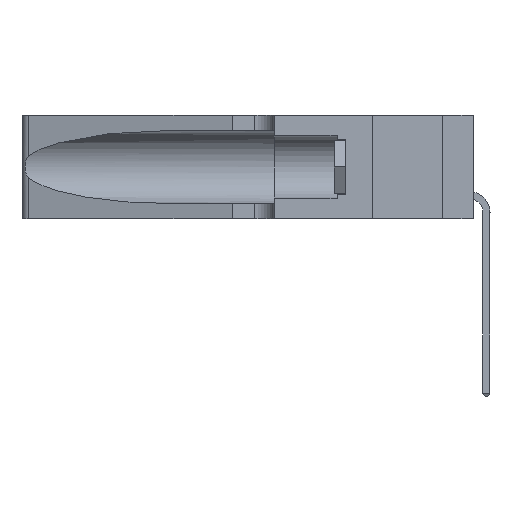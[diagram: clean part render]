
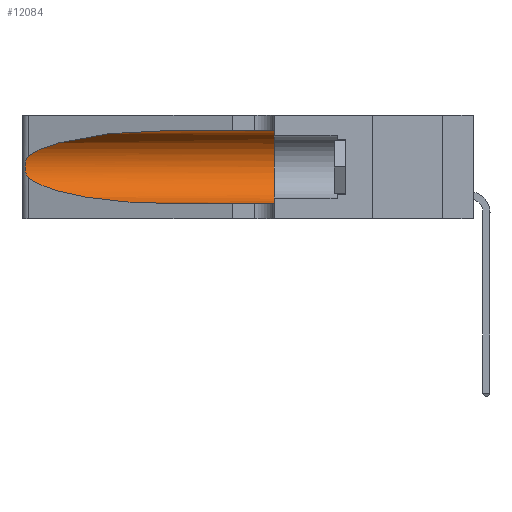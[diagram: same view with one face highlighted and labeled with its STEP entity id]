
A CAD part, left-side view. The second image highlights one B-rep face of the part: STEP entity #12084.
In plain terms, the highlighted cylindrical face has radius 3.308 mm (diameter 6.617 mm), a partial arc.
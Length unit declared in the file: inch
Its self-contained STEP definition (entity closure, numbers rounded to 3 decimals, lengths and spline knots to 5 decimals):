
#954 = CARTESIAN_POINT ( 'NONE',  ( 0.1305, 0.35, 0.185 ) ) ;
#1861 = EDGE_CURVE ( 'NONE', #3503, #39912, #5490, .T. ) ;
#1946 = VECTOR ( 'NONE', #24307, 39.37008 ) ;
#3069 = LINE ( 'NONE', #7002, #38445 ) ;
#3237 = VERTEX_POINT ( 'NONE', #25100 ) ;
#3428 = EDGE_CURVE ( 'NONE', #3237, #4760, #23144, .T. ) ;
#3503 = VERTEX_POINT ( 'NONE', #21320 ) ;
#4322 = AXIS2_PLACEMENT_3D ( 'NONE', #46529, #43051, #35353 ) ;
#4760 = VERTEX_POINT ( 'NONE', #31381 ) ;
#4955 = ORIENTED_EDGE ( 'NONE', *, *, #37876, .T. ) ;
#4978 = EDGE_CURVE ( 'NONE', #3503, #3237, #3069, .T. ) ;
#5490 =( BOUNDED_CURVE ( )  B_SPLINE_CURVE ( 3, ( #45179, #5866, #49540, #33863 ),
 .UNSPECIFIED., .F., .T. ) 
 B_SPLINE_CURVE_WITH_KNOTS ( ( 4, 4 ),
 ( 1.5708, 2.84003 ),
 .UNSPECIFIED. ) 
 CURVE ( )  GEOMETRIC_REPRESENTATION_ITEM ( )  RATIONAL_B_SPLINE_CURVE ( ( 1., 0.87, 0.87, 1. ) ) 
 REPRESENTATION_ITEM ( '' )  );
#5866 = CARTESIAN_POINT ( 'NONE',  ( 0.18966, 0.96281, 0.31525 ) ) ;
#6315 = CARTESIAN_POINT ( 'NONE',  ( 0.1305, 0.72297, 0.05475 ) ) ;
#6815 = CARTESIAN_POINT ( 'NONE',  ( 0.26075, 1.23896, 0.19203 ) ) ;
#7002 = CARTESIAN_POINT ( 'NONE',  ( 0.1305, 1.61858, 0.31525 ) ) ;
#8312 = EDGE_CURVE ( 'NONE', #39912, #24991, #38665, .T. ) ;
#10806 = CARTESIAN_POINT ( 'NONE',  ( 0.25487, 1.22718, 0.22369 ) ) ;
#10985 = CARTESIAN_POINT ( 'NONE',  ( 0.25854, 1.2359, 0.20912 ) ) ;
#12084 = ADVANCED_FACE ( 'NONE', ( #42642 ), #25212, .F. ) ;
#12540 = LINE ( 'NONE', #28469, #1946 ) ;
#13030 = AXIS2_PLACEMENT_3D ( 'NONE', #954, #40420, #17020 ) ;
#14125 = CARTESIAN_POINT ( 'NONE',  ( 0.25487, 1.22718, 0.14631 ) ) ;
#14796 = CARTESIAN_POINT ( 'NONE',  ( 0.25787, 1.23484, 0.2124 ) ) ;
#16387 = ORIENTED_EDGE ( 'NONE', *, *, #1861, .T. ) ;
#17020 = DIRECTION ( 'NONE',  ( 0., 0., 1. ) ) ;
#18325 = CARTESIAN_POINT ( 'NONE',  ( 0.2373, 1.15595, 0.08982 ) ) ;
#18797 = CARTESIAN_POINT ( 'NONE',  ( 0.25856, 1.23593, 0.16098 ) ) ;
#18806 = ORIENTED_EDGE ( 'NONE', *, *, #35010, .T. ) ;
#21320 = CARTESIAN_POINT ( 'NONE',  ( 0.1305, 0.72297, 0.31525 ) ) ;
#21759 = CARTESIAN_POINT ( 'NONE',  ( 0.25487, 1.22718, 0.14631 ) ) ;
#22218 = CARTESIAN_POINT ( 'NONE',  ( 0.25789, 1.23486, 0.15765 ) ) ;
#23144 = CIRCLE ( 'NONE', #13030, 0.13025 ) ;
#24307 = DIRECTION ( 'NONE',  ( 0., -1., 0. ) ) ;
#24991 = VERTEX_POINT ( 'NONE', #14125 ) ;
#25100 = CARTESIAN_POINT ( 'NONE',  ( 0.1305, 0.35, 0.31525 ) ) ;
#25212 = CYLINDRICAL_SURFACE ( 'NONE', #4322, 0.13025 ) ;
#25939 = CARTESIAN_POINT ( 'NONE',  ( 0.18966, 0.96281, 0.05475 ) ) ;
#26661 = DIRECTION ( 'NONE',  ( 0., -1., 0. ) ) ;
#26987 = EDGE_LOOP ( 'NONE', ( #16387, #29256, #4955, #18806, #27594, #30817 ) ) ;
#27594 = ORIENTED_EDGE ( 'NONE', *, *, #3428, .F. ) ;
#28469 = CARTESIAN_POINT ( 'NONE',  ( 0.1305, 1.61858, 0.05475 ) ) ;
#29256 = ORIENTED_EDGE ( 'NONE', *, *, #8312, .T. ) ;
#29987 = CARTESIAN_POINT ( 'NONE',  ( 0.1305, 0.72297, 0.05475 ) ) ;
#30817 = ORIENTED_EDGE ( 'NONE', *, *, #4978, .F. ) ;
#31381 = CARTESIAN_POINT ( 'NONE',  ( 0.1305, 0.35, 0.05475 ) ) ;
#33863 = CARTESIAN_POINT ( 'NONE',  ( 0.25487, 1.22718, 0.22369 ) ) ;
#33900 =( BOUNDED_CURVE ( )  B_SPLINE_CURVE ( 3, ( #21759, #18325, #25939, #29987 ),
 .UNSPECIFIED., .F., .F. ) 
 B_SPLINE_CURVE_WITH_KNOTS ( ( 4, 4 ),
 ( 3.44316, 4.71239 ),
 .UNSPECIFIED. ) 
 CURVE ( )  GEOMETRIC_REPRESENTATION_ITEM ( )  RATIONAL_B_SPLINE_CURVE ( ( 1., 0.87, 0.87, 1. ) ) 
 REPRESENTATION_ITEM ( '' )  );
#34408 = CARTESIAN_POINT ( 'NONE',  ( 0.26018, 1.23835, 0.19895 ) ) ;
#35010 = EDGE_CURVE ( 'NONE', #37280, #4760, #12540, .T. ) ;
#35353 = DIRECTION ( 'NONE',  ( 0., 0., -1. ) ) ;
#37280 = VERTEX_POINT ( 'NONE', #6315 ) ;
#37876 = EDGE_CURVE ( 'NONE', #24991, #37280, #33900, .T. ) ;
#38445 = VECTOR ( 'NONE', #26661, 39.37008 ) ;
#38535 = CARTESIAN_POINT ( 'NONE',  ( 0.25639, 1.23184, 0.21858 ) ) ;
#38665 = B_SPLINE_CURVE_WITH_KNOTS ( 'NONE', 3,
 ( #10806, #42652, #38535, #14796, #10985, #34408, #6815, #38709, #45933, #18797, #22218, #42292, #46116, #49898 ),
 .UNSPECIFIED., .F., .F.,
 ( 4, 2, 2, 2, 2, 2, 4 ),
 ( 0., 0.00027, 0.00053, 0.00107, 0.0016, 0.00187, 0.00214 ),
 .UNSPECIFIED. ) ;
#38709 = CARTESIAN_POINT ( 'NONE',  ( 0.26075, 1.23896, 0.178 ) ) ;
#39912 = VERTEX_POINT ( 'NONE', #41609 ) ;
#40420 = DIRECTION ( 'NONE',  ( 0., 1., 0. ) ) ;
#41609 = CARTESIAN_POINT ( 'NONE',  ( 0.25487, 1.22718, 0.22369 ) ) ;
#42292 = CARTESIAN_POINT ( 'NONE',  ( 0.25639, 1.23186, 0.15144 ) ) ;
#42642 = FACE_OUTER_BOUND ( 'NONE', #26987, .T. ) ;
#42652 = CARTESIAN_POINT ( 'NONE',  ( 0.25555, 1.22994, 0.2215 ) ) ;
#43051 = DIRECTION ( 'NONE',  ( 0., -1., 0. ) ) ;
#45179 = CARTESIAN_POINT ( 'NONE',  ( 0.1305, 0.72297, 0.31525 ) ) ;
#45933 = CARTESIAN_POINT ( 'NONE',  ( 0.26017, 1.23833, 0.17102 ) ) ;
#46116 = CARTESIAN_POINT ( 'NONE',  ( 0.25555, 1.22993, 0.14849 ) ) ;
#46529 = CARTESIAN_POINT ( 'NONE',  ( 0.1305, 1.61858, 0.185 ) ) ;
#49540 = CARTESIAN_POINT ( 'NONE',  ( 0.2373, 1.15595, 0.28018 ) ) ;
#49898 = CARTESIAN_POINT ( 'NONE',  ( 0.25487, 1.22718, 0.14631 ) ) ;
